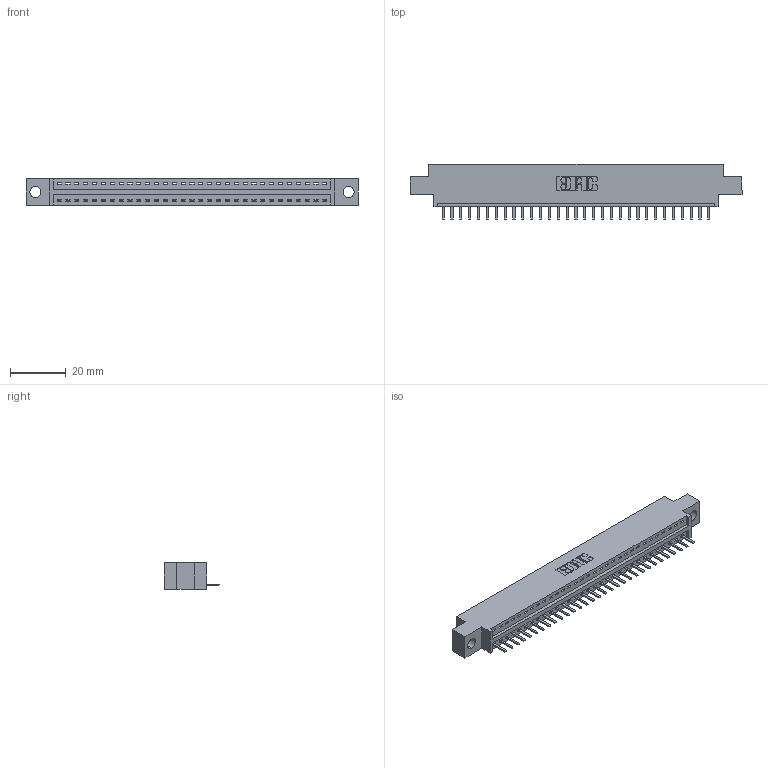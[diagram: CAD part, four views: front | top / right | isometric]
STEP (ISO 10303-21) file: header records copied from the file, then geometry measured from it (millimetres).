
FILE_DESCRIPTION (( 'STEP AP203' ), '1' );
FILE_NAME ('396-031-520-604.STEP', '2018-09-05T08:31:07', ( '' ), ( '' ), 'SwSTEP 2.0', 'SolidWorks 2016', '' );
FILE_SCHEMA (( 'CONFIG_CONTROL_DESIGN' ));
Length unit declared in the file: inch
Products named in the file (3): 345-292-001_345-293-120; 396-031-520-604; 346 Part_0.170 Offset - 0.156 Dia-TH
Assembly tree (32 placements, depth 2):
  396-031-520-604
    346 Part_0.170 Offset - 0.156 Dia-TH
    345-292-001_345-293-120  x31
Bounding box: 119 x 20.02 x 9.4 mm (x, y, z)
Volume: 10983.4 mm3; surface area: 13276.8 mm2
Topology: 32 solids, 32 shells, 2048 faces, 6045 edges, 3946 vertices
Faces by surface type: plane 1382, cylinder 666
Entity records: 20969 total; most frequent: CARTESIAN_POINT 3617, ORIENTED_EDGE 3570, DIRECTION 3191, EDGE_CURVE 1785, LINE 1525, VECTOR 1525, VERTEX_POINT 1186, AXIS2_PLACEMENT_3D 833
